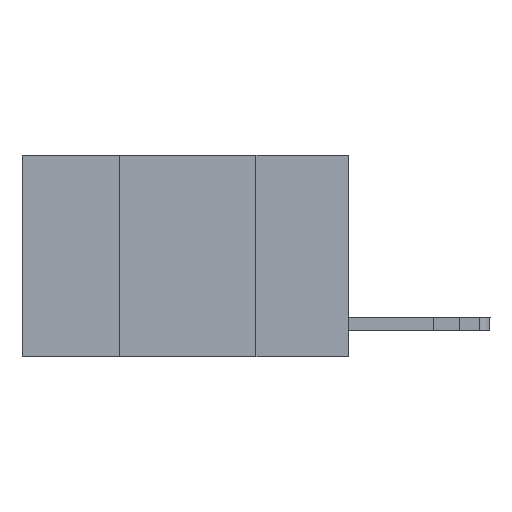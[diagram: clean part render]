
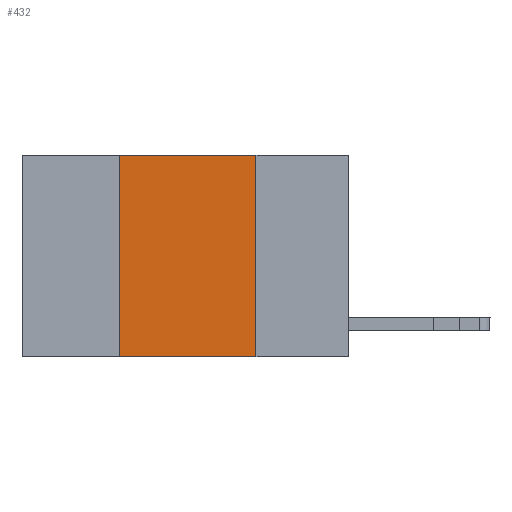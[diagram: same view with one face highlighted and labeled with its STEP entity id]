
A CAD part, left-side view. The second image highlights one B-rep face of the part: STEP entity #432.
In plain terms, the highlighted planar face has unit normal (-1, 0, 0).
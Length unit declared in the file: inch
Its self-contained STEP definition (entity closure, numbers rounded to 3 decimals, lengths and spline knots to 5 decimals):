
#432 = ADVANCED_FACE ( 'NONE', ( #1031 ), #7929, .F. ) ;
#510 = ORIENTED_EDGE ( 'NONE', *, *, #620, .F. ) ;
#620 = EDGE_CURVE ( 'NONE', #13072, #8848, #1464, .T. ) ;
#1031 = FACE_OUTER_BOUND ( 'NONE', #1153, .T. ) ;
#1153 = EDGE_LOOP ( 'NONE', ( #17198, #16838, #510, #6067 ) ) ;
#1308 = CARTESIAN_POINT ( 'NONE',  ( 0., 0.42, 0. ) ) ;
#1464 = LINE ( 'NONE', #7180, #10729 ) ;
#1512 = DIRECTION ( 'NONE',  ( 0., -1., 0. ) ) ;
#2629 = VECTOR ( 'NONE', #1512, 39.37008 ) ;
#2970 = VECTOR ( 'NONE', #15916, 39.37008 ) ;
#3958 = VERTEX_POINT ( 'NONE', #5492 ) ;
#3963 = EDGE_CURVE ( 'NONE', #8848, #11265, #16455, .T. ) ;
#4077 = AXIS2_PLACEMENT_3D ( 'NONE', #13344, #5197, #15054 ) ;
#4668 = VECTOR ( 'NONE', #11701, 39.37008 ) ;
#4865 = CARTESIAN_POINT ( 'NONE',  ( 0., 0.6, -0.37 ) ) ;
#5045 = EDGE_CURVE ( 'NONE', #11265, #3958, #14589, .T. ) ;
#5197 = DIRECTION ( 'NONE',  ( 1., 0., 0. ) ) ;
#5415 = EDGE_CURVE ( 'NONE', #13072, #3958, #17260, .T. ) ;
#5492 = CARTESIAN_POINT ( 'NONE',  ( 0., 0.17, -0.37 ) ) ;
#6067 = ORIENTED_EDGE ( 'NONE', *, *, #5415, .T. ) ;
#7180 = CARTESIAN_POINT ( 'NONE',  ( 0., 0.42, 0. ) ) ;
#7929 = PLANE ( 'NONE',  #4077 ) ;
#8749 = CARTESIAN_POINT ( 'NONE',  ( 0., 0.17, 0. ) ) ;
#8848 = VERTEX_POINT ( 'NONE', #1308 ) ;
#9161 = CARTESIAN_POINT ( 'NONE',  ( 0., 0.42, -0.37 ) ) ;
#9598 = CARTESIAN_POINT ( 'NONE',  ( 0., 0.6, 0. ) ) ;
#10729 = VECTOR ( 'NONE', #15324, 39.37008 ) ;
#11265 = VERTEX_POINT ( 'NONE', #8749 ) ;
#11701 = DIRECTION ( 'NONE',  ( 0., 0., -1. ) ) ;
#13072 = VERTEX_POINT ( 'NONE', #9161 ) ;
#13344 = CARTESIAN_POINT ( 'NONE',  ( 0., 0.6, 0. ) ) ;
#14502 = CARTESIAN_POINT ( 'NONE',  ( 0., 0.17, 0. ) ) ;
#14589 = LINE ( 'NONE', #14502, #4668 ) ;
#15054 = DIRECTION ( 'NONE',  ( 0., 0., -1. ) ) ;
#15324 = DIRECTION ( 'NONE',  ( 0., 0., 1. ) ) ;
#15916 = DIRECTION ( 'NONE',  ( 0., -1., 0. ) ) ;
#16455 = LINE ( 'NONE', #9598, #2629 ) ;
#16838 = ORIENTED_EDGE ( 'NONE', *, *, #3963, .F. ) ;
#17198 = ORIENTED_EDGE ( 'NONE', *, *, #5045, .F. ) ;
#17260 = LINE ( 'NONE', #4865, #2970 ) ;
